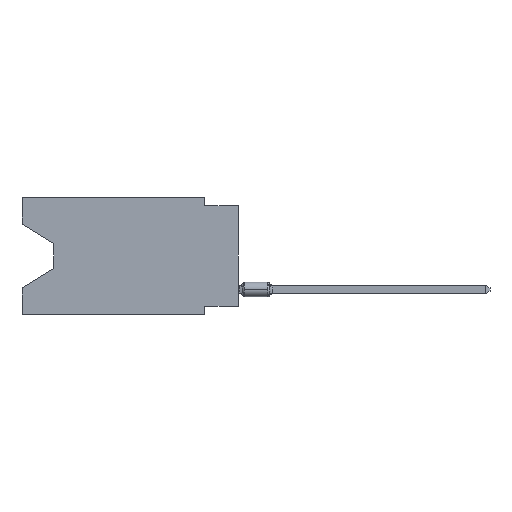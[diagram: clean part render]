
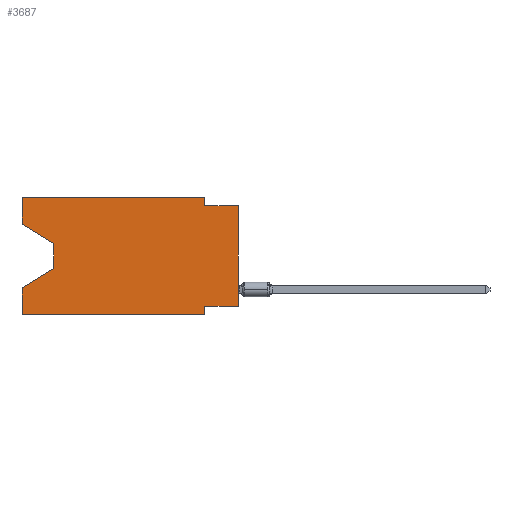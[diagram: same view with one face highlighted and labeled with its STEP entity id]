
A CAD part, left-side view. The second image highlights one B-rep face of the part: STEP entity #3687.
In plain terms, the highlighted planar face has unit normal (-1, 0, 0).
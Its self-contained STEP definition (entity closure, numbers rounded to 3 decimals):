
#8 = CARTESIAN_POINT ( 'NONE',  ( 0., 13.97, -5.385 ) ) ;
#67 = VERTEX_POINT ( 'NONE', #13312 ) ;
#170 = DIRECTION ( 'NONE',  ( 0., -1., 0. ) ) ;
#453 = CARTESIAN_POINT ( 'NONE',  ( 0., 16.383, 0. ) ) ;
#640 = EDGE_CURVE ( 'NONE', #5996, #9796, #1463, .T. ) ;
#813 = LINE ( 'NONE', #8693, #2860 ) ;
#981 = CARTESIAN_POINT ( 'NONE',  ( 0., 0., -8.255 ) ) ;
#1052 = DIRECTION ( 'NONE',  ( 0., 0.855, -0.519 ) ) ;
#1340 = CARTESIAN_POINT ( 'NONE',  ( 0., 16.383, 0. ) ) ;
#1463 = LINE ( 'NONE', #9414, #7409 ) ;
#1663 = DIRECTION ( 'NONE',  ( 0., 0., -1. ) ) ;
#1698 = ORIENTED_EDGE ( 'NONE', *, *, #6037, .T. ) ;
#1832 = CARTESIAN_POINT ( 'NONE',  ( 0., 2.54, 0. ) ) ;
#2188 = ORIENTED_EDGE ( 'NONE', *, *, #12596, .F. ) ;
#2302 = VECTOR ( 'NONE', #170, 1000. ) ;
#2403 = LINE ( 'NONE', #8, #3906 ) ;
#2432 = CARTESIAN_POINT ( 'NONE',  ( 0., 0., 0. ) ) ;
#2462 = LINE ( 'NONE', #1340, #7049 ) ;
#2860 = VECTOR ( 'NONE', #14427, 1000. ) ;
#2916 = EDGE_CURVE ( 'NONE', #67, #11595, #11316, .T. ) ;
#2995 = ORIENTED_EDGE ( 'NONE', *, *, #9910, .F. ) ;
#3225 = ORIENTED_EDGE ( 'NONE', *, *, #2916, .T. ) ;
#3433 = DIRECTION ( 'NONE',  ( 0., 0., -1. ) ) ;
#3519 = ORIENTED_EDGE ( 'NONE', *, *, #9670, .F. ) ;
#3687 = ADVANCED_FACE ( 'NONE', ( #10903 ), #5181, .F. ) ;
#3821 = DIRECTION ( 'NONE',  ( 0., -0.855, -0.519 ) ) ;
#3890 = LINE ( 'NONE', #10453, #2302 ) ;
#3906 = VECTOR ( 'NONE', #1052, 1000. ) ;
#4758 = VERTEX_POINT ( 'NONE', #6929 ) ;
#4936 = DIRECTION ( 'NONE',  ( 0., 0., 1. ) ) ;
#5020 = DIRECTION ( 'NONE',  ( 0., 0., 1. ) ) ;
#5181 = PLANE ( 'NONE',  #13613 ) ;
#5322 = DIRECTION ( 'NONE',  ( 0., 0., -1. ) ) ;
#5440 = VECTOR ( 'NONE', #3821, 1000. ) ;
#5492 = VERTEX_POINT ( 'NONE', #14034 ) ;
#5996 = VERTEX_POINT ( 'NONE', #8069 ) ;
#6037 = EDGE_CURVE ( 'NONE', #8119, #9533, #9266, .T. ) ;
#6391 = EDGE_LOOP ( 'NONE', ( #11706, #9131, #14456, #10761, #3225, #2995, #2188, #1698, #10597, #9860, #10088, #3519 ) ) ;
#6836 = VECTOR ( 'NONE', #9279, 1000. ) ;
#6929 = CARTESIAN_POINT ( 'NONE',  ( 0., 16.383, -2.038 ) ) ;
#7049 = VECTOR ( 'NONE', #4936, 1000. ) ;
#7060 = CARTESIAN_POINT ( 'NONE',  ( 0., 0., -0.635 ) ) ;
#7084 = DIRECTION ( 'NONE',  ( 0., 0., -1. ) ) ;
#7372 = VERTEX_POINT ( 'NONE', #13099 ) ;
#7409 = VECTOR ( 'NONE', #7084, 1000. ) ;
#7804 = LINE ( 'NONE', #13221, #13545 ) ;
#7823 = EDGE_CURVE ( 'NONE', #4758, #5996, #10670, .T. ) ;
#7856 = EDGE_CURVE ( 'NONE', #5492, #14557, #3890, .T. ) ;
#7956 = CARTESIAN_POINT ( 'NONE',  ( 0., 2.54, -8.89 ) ) ;
#8069 = CARTESIAN_POINT ( 'NONE',  ( 0., 13.97, -3.505 ) ) ;
#8119 = VERTEX_POINT ( 'NONE', #981 ) ;
#8131 = LINE ( 'NONE', #7060, #12024 ) ;
#8226 = CARTESIAN_POINT ( 'NONE',  ( 0., 2.54, -8.89 ) ) ;
#8693 = CARTESIAN_POINT ( 'NONE',  ( 0., 0., -8.255 ) ) ;
#9004 = CARTESIAN_POINT ( 'NONE',  ( 0., 16.383, 0. ) ) ;
#9055 = DIRECTION ( 'NONE',  ( 0., 0., 1. ) ) ;
#9116 = CARTESIAN_POINT ( 'NONE',  ( 0., 2.54, -8.255 ) ) ;
#9131 = ORIENTED_EDGE ( 'NONE', *, *, #640, .T. ) ;
#9203 = VECTOR ( 'NONE', #5020, 1000. ) ;
#9213 = VECTOR ( 'NONE', #3433, 1000. ) ;
#9244 = CARTESIAN_POINT ( 'NONE',  ( 0., 0., -0.635 ) ) ;
#9266 = LINE ( 'NONE', #2432, #13128 ) ;
#9279 = DIRECTION ( 'NONE',  ( 0., -1., 0. ) ) ;
#9414 = CARTESIAN_POINT ( 'NONE',  ( 0., 13.97, -3.505 ) ) ;
#9533 = VERTEX_POINT ( 'NONE', #9244 ) ;
#9670 = EDGE_CURVE ( 'NONE', #4758, #5492, #12768, .T. ) ;
#9700 = DIRECTION ( 'NONE',  ( 1., 0., 0. ) ) ;
#9796 = VERTEX_POINT ( 'NONE', #12242 ) ;
#9852 = VERTEX_POINT ( 'NONE', #12168 ) ;
#9860 = ORIENTED_EDGE ( 'NONE', *, *, #11097, .F. ) ;
#9910 = EDGE_CURVE ( 'NONE', #14785, #11595, #12541, .T. ) ;
#10088 = ORIENTED_EDGE ( 'NONE', *, *, #7856, .F. ) ;
#10453 = CARTESIAN_POINT ( 'NONE',  ( 0., 16.383, 0. ) ) ;
#10596 = DIRECTION ( 'NONE',  ( 0., -1., 0. ) ) ;
#10597 = ORIENTED_EDGE ( 'NONE', *, *, #14764, .F. ) ;
#10670 = LINE ( 'NONE', #13923, #5440 ) ;
#10761 = ORIENTED_EDGE ( 'NONE', *, *, #11301, .F. ) ;
#10903 = FACE_OUTER_BOUND ( 'NONE', #6391, .T. ) ;
#11097 = EDGE_CURVE ( 'NONE', #14557, #9852, #7804, .T. ) ;
#11301 = EDGE_CURVE ( 'NONE', #67, #7372, #2462, .T. ) ;
#11316 = LINE ( 'NONE', #13730, #6836 ) ;
#11595 = VERTEX_POINT ( 'NONE', #8226 ) ;
#11706 = ORIENTED_EDGE ( 'NONE', *, *, #7823, .T. ) ;
#12024 = VECTOR ( 'NONE', #10596, 1000. ) ;
#12168 = CARTESIAN_POINT ( 'NONE',  ( 0., 2.54, -0.635 ) ) ;
#12242 = CARTESIAN_POINT ( 'NONE',  ( 0., 13.97, -5.385 ) ) ;
#12294 = EDGE_CURVE ( 'NONE', #9796, #7372, #2403, .T. ) ;
#12541 = LINE ( 'NONE', #7956, #9213 ) ;
#12596 = EDGE_CURVE ( 'NONE', #8119, #14785, #813, .T. ) ;
#12768 = LINE ( 'NONE', #453, #9203 ) ;
#13099 = CARTESIAN_POINT ( 'NONE',  ( 0., 16.383, -6.852 ) ) ;
#13128 = VECTOR ( 'NONE', #9055, 1000. ) ;
#13221 = CARTESIAN_POINT ( 'NONE',  ( 0., 2.54, 0. ) ) ;
#13312 = CARTESIAN_POINT ( 'NONE',  ( 0., 16.383, -8.89 ) ) ;
#13545 = VECTOR ( 'NONE', #5322, 1000. ) ;
#13613 = AXIS2_PLACEMENT_3D ( 'NONE', #9004, #9700, #1663 ) ;
#13730 = CARTESIAN_POINT ( 'NONE',  ( 0., 16.383, -8.89 ) ) ;
#13923 = CARTESIAN_POINT ( 'NONE',  ( 0., 16.383, -2.038 ) ) ;
#14034 = CARTESIAN_POINT ( 'NONE',  ( 0., 16.383, 0. ) ) ;
#14427 = DIRECTION ( 'NONE',  ( 0., 1., 0. ) ) ;
#14456 = ORIENTED_EDGE ( 'NONE', *, *, #12294, .T. ) ;
#14557 = VERTEX_POINT ( 'NONE', #1832 ) ;
#14764 = EDGE_CURVE ( 'NONE', #9852, #9533, #8131, .T. ) ;
#14785 = VERTEX_POINT ( 'NONE', #9116 ) ;
